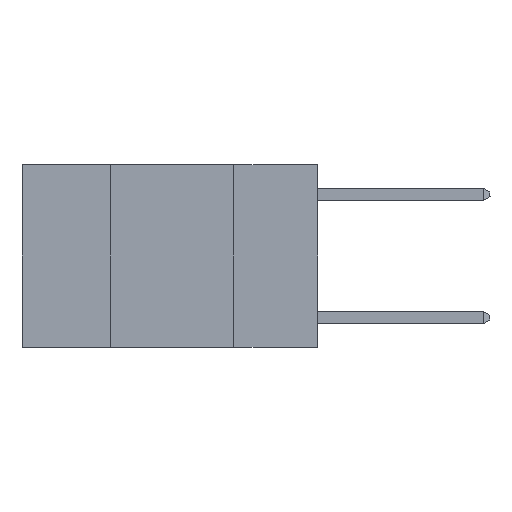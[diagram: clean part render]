
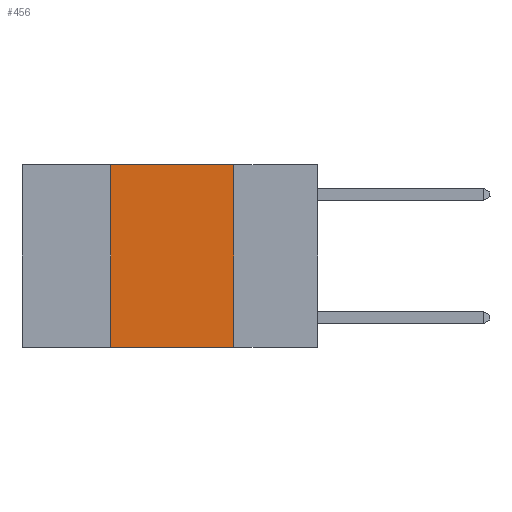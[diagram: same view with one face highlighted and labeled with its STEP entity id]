
A CAD part, left-side view. The second image highlights one B-rep face of the part: STEP entity #456.
In plain terms, the highlighted planar face has unit normal (-1, 0, 0).
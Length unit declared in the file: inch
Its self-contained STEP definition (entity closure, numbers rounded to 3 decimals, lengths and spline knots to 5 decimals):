
#399 = CARTESIAN_POINT ( 'NONE',  ( 0., 0.17, 0. ) ) ;
#456 = ADVANCED_FACE ( 'NONE', ( #3069 ), #1360, .F. ) ;
#537 = VECTOR ( 'NONE', #7116, 39.37008 ) ;
#570 = ORIENTED_EDGE ( 'NONE', *, *, #8519, .T. ) ;
#657 = CARTESIAN_POINT ( 'NONE',  ( 0., 0.17, -0.37 ) ) ;
#696 = DIRECTION ( 'NONE',  ( 0., -1., 0. ) ) ;
#943 = ORIENTED_EDGE ( 'NONE', *, *, #10491, .F. ) ;
#1179 = CARTESIAN_POINT ( 'NONE',  ( 0., 0.42, -0.37 ) ) ;
#1245 = VECTOR ( 'NONE', #1991, 39.37008 ) ;
#1360 = PLANE ( 'NONE',  #2955 ) ;
#1590 = EDGE_LOOP ( 'NONE', ( #2478, #943, #9076, #570 ) ) ;
#1991 = DIRECTION ( 'NONE',  ( 0., 0., -1. ) ) ;
#2057 = LINE ( 'NONE', #7052, #1245 ) ;
#2478 = ORIENTED_EDGE ( 'NONE', *, *, #9638, .F. ) ;
#2628 = EDGE_CURVE ( 'NONE', #6557, #6489, #10165, .T. ) ;
#2955 = AXIS2_PLACEMENT_3D ( 'NONE', #4912, #8345, #8229 ) ;
#3069 = FACE_OUTER_BOUND ( 'NONE', #1590, .T. ) ;
#3268 = CARTESIAN_POINT ( 'NONE',  ( 0., 0.42, 0. ) ) ;
#4640 = CARTESIAN_POINT ( 'NONE',  ( 0., 0.6, 0. ) ) ;
#4912 = CARTESIAN_POINT ( 'NONE',  ( 0., 0.6, 0. ) ) ;
#5965 = CARTESIAN_POINT ( 'NONE',  ( 0., 0.6, -0.37 ) ) ;
#6120 = VECTOR ( 'NONE', #6857, 39.37008 ) ;
#6489 = VERTEX_POINT ( 'NONE', #6978 ) ;
#6557 = VERTEX_POINT ( 'NONE', #1179 ) ;
#6857 = DIRECTION ( 'NONE',  ( 0., 0., 1. ) ) ;
#6978 = CARTESIAN_POINT ( 'NONE',  ( 0., 0.42, 0. ) ) ;
#7052 = CARTESIAN_POINT ( 'NONE',  ( 0., 0.17, 0. ) ) ;
#7116 = DIRECTION ( 'NONE',  ( 0., -1., 0. ) ) ;
#8229 = DIRECTION ( 'NONE',  ( 0., 0., -1. ) ) ;
#8345 = DIRECTION ( 'NONE',  ( 1., 0., 0. ) ) ;
#8519 = EDGE_CURVE ( 'NONE', #6557, #11034, #10209, .T. ) ;
#8789 = VERTEX_POINT ( 'NONE', #399 ) ;
#8791 = VECTOR ( 'NONE', #696, 39.37008 ) ;
#8974 = LINE ( 'NONE', #4640, #537 ) ;
#9076 = ORIENTED_EDGE ( 'NONE', *, *, #2628, .F. ) ;
#9638 = EDGE_CURVE ( 'NONE', #8789, #11034, #2057, .T. ) ;
#10165 = LINE ( 'NONE', #3268, #6120 ) ;
#10209 = LINE ( 'NONE', #5965, #8791 ) ;
#10491 = EDGE_CURVE ( 'NONE', #6489, #8789, #8974, .T. ) ;
#11034 = VERTEX_POINT ( 'NONE', #657 ) ;
